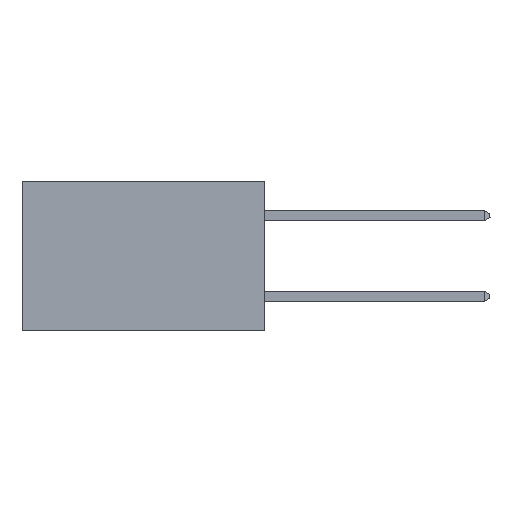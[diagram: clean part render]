
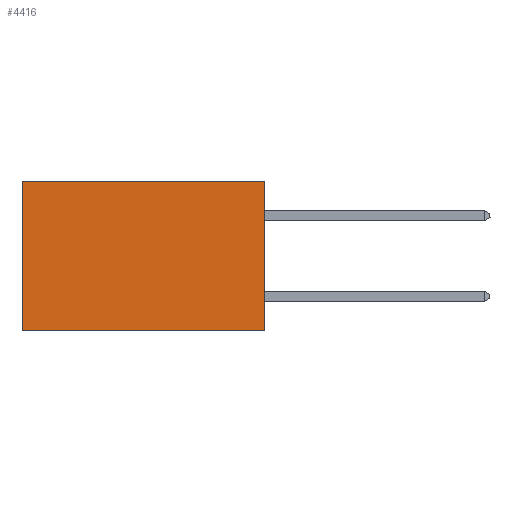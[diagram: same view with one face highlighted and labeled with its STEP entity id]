
A CAD part, left-side view. The second image highlights one B-rep face of the part: STEP entity #4416.
In plain terms, the highlighted planar face has unit normal (-1, 0, 0).
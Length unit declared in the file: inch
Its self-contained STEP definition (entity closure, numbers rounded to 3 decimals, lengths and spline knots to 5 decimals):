
#845 = CARTESIAN_POINT ( 'NONE',  ( 0.298, 0., 0. ) ) ;
#1144 = LINE ( 'NONE', #845, #7949 ) ;
#1542 = VECTOR ( 'NONE', #12972, 39.37008 ) ;
#2110 = VERTEX_POINT ( 'NONE', #7730 ) ;
#2498 = CARTESIAN_POINT ( 'NONE',  ( 0.298, 0., -0.37 ) ) ;
#3051 = VERTEX_POINT ( 'NONE', #11968 ) ;
#3169 = DIRECTION ( 'NONE',  ( 0., 1., 0. ) ) ;
#3956 = CARTESIAN_POINT ( 'NONE',  ( 0.298, 0.6, -0.37 ) ) ;
#4317 = CARTESIAN_POINT ( 'NONE',  ( 0.298, 0., 0. ) ) ;
#4334 = EDGE_CURVE ( 'NONE', #3051, #12383, #11819, .T. ) ;
#4413 = DIRECTION ( 'NONE',  ( 0., 1., 0. ) ) ;
#4416 = ADVANCED_FACE ( 'NONE', ( #9595 ), #5662, .F. ) ;
#4889 = ORIENTED_EDGE ( 'NONE', *, *, #6474, .F. ) ;
#5248 = ORIENTED_EDGE ( 'NONE', *, *, #4334, .T. ) ;
#5356 = EDGE_CURVE ( 'NONE', #8113, #12383, #6811, .T. ) ;
#5662 = PLANE ( 'NONE',  #12197 ) ;
#5967 = VECTOR ( 'NONE', #4413, 39.37008 ) ;
#6357 = VECTOR ( 'NONE', #3169, 39.37008 ) ;
#6457 = DIRECTION ( 'NONE',  ( 0., 0., -1. ) ) ;
#6474 = EDGE_CURVE ( 'NONE', #2110, #8113, #1144, .T. ) ;
#6568 = CARTESIAN_POINT ( 'NONE',  ( 0.298, 0., -0.37 ) ) ;
#6732 = DIRECTION ( 'NONE',  ( 1., 0., 0. ) ) ;
#6811 = LINE ( 'NONE', #6568, #5967 ) ;
#7730 = CARTESIAN_POINT ( 'NONE',  ( 0.298, 0., 0. ) ) ;
#7949 = VECTOR ( 'NONE', #6457, 39.37008 ) ;
#7985 = EDGE_LOOP ( 'NONE', ( #5248, #10771, #4889, #10255 ) ) ;
#8113 = VERTEX_POINT ( 'NONE', #2498 ) ;
#8481 = EDGE_CURVE ( 'NONE', #2110, #3051, #12358, .T. ) ;
#9595 = FACE_OUTER_BOUND ( 'NONE', #7985, .T. ) ;
#9661 = CARTESIAN_POINT ( 'NONE',  ( 0.298, 0.6, 0. ) ) ;
#9990 = DIRECTION ( 'NONE',  ( 0., 0., -1. ) ) ;
#10042 = CARTESIAN_POINT ( 'NONE',  ( 0.298, 0., 0. ) ) ;
#10255 = ORIENTED_EDGE ( 'NONE', *, *, #8481, .T. ) ;
#10771 = ORIENTED_EDGE ( 'NONE', *, *, #5356, .F. ) ;
#11819 = LINE ( 'NONE', #9661, #1542 ) ;
#11968 = CARTESIAN_POINT ( 'NONE',  ( 0.298, 0.6, 0. ) ) ;
#12197 = AXIS2_PLACEMENT_3D ( 'NONE', #10042, #6732, #9990 ) ;
#12358 = LINE ( 'NONE', #4317, #6357 ) ;
#12383 = VERTEX_POINT ( 'NONE', #3956 ) ;
#12972 = DIRECTION ( 'NONE',  ( 0., 0., -1. ) ) ;
